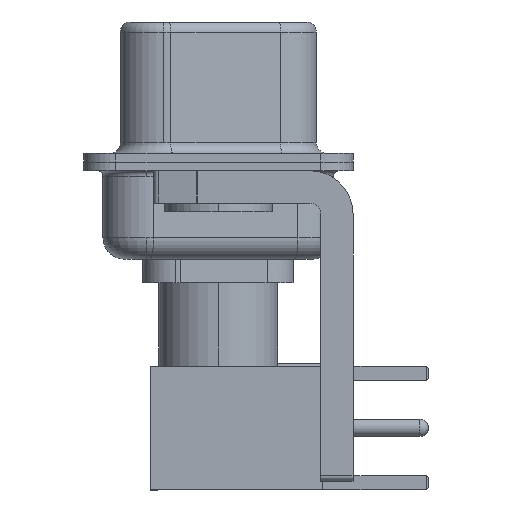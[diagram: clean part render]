
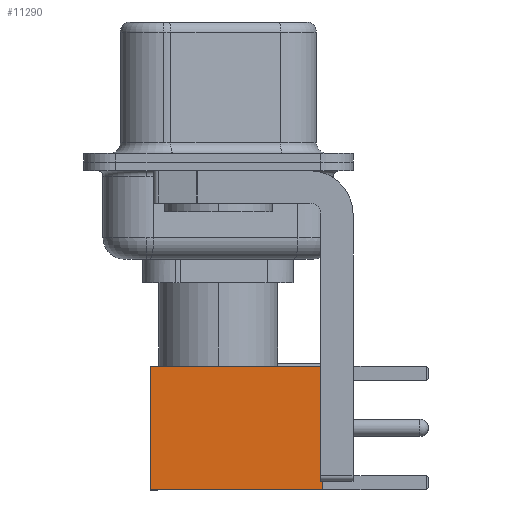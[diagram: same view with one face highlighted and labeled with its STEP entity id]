
A CAD part, left-side view. The second image highlights one B-rep face of the part: STEP entity #11290.
In plain terms, the highlighted face is planar.
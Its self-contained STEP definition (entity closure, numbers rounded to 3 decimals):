
#524 = CARTESIAN_POINT ( 'NONE',  ( 0., 2.875, 8. ) ) ;
#756 = EDGE_CURVE ( 'NONE', #16886, #11554, #18207, .T. ) ;
#2375 = AXIS2_PLACEMENT_3D ( 'NONE', #16512, #8999, #18196 ) ;
#4478 = PLANE ( 'NONE',  #2375 ) ;
#4785 = CARTESIAN_POINT ( 'NONE',  ( -2.875, 2.875, 0. ) ) ;
#5215 = LINE ( 'NONE', #524, #28348 ) ;
#5266 = CARTESIAN_POINT ( 'NONE',  ( 2.875, 2.875, 0. ) ) ;
#6453 = EDGE_CURVE ( 'NONE', #27923, #16886, #5215, .T. ) ;
#6469 = VECTOR ( 'NONE', #14105, 1000. ) ;
#7337 = FACE_OUTER_BOUND ( 'NONE', #20268, .T. ) ;
#8255 = CARTESIAN_POINT ( 'NONE',  ( 0., 2.875, 0. ) ) ;
#8999 = DIRECTION ( 'NONE',  ( 0., 1., 0. ) ) ;
#10598 = VECTOR ( 'NONE', #17143, 1000. ) ;
#11284 = VERTEX_POINT ( 'NONE', #20448 ) ;
#11290 = ADVANCED_FACE ( 'NONE', ( #7337 ), #4478, .T. ) ;
#11554 = VERTEX_POINT ( 'NONE', #23455 ) ;
#11749 = DIRECTION ( 'NONE',  ( 0., 0., -1. ) ) ;
#12223 = EDGE_CURVE ( 'NONE', #11284, #11554, #12325, .T. ) ;
#12325 = LINE ( 'NONE', #8255, #10598 ) ;
#14105 = DIRECTION ( 'NONE',  ( 0., 0., -1. ) ) ;
#14378 = DIRECTION ( 'NONE',  ( -1., 0., 0. ) ) ;
#16512 = CARTESIAN_POINT ( 'NONE',  ( 2.875, 2.875, 0. ) ) ;
#16886 = VERTEX_POINT ( 'NONE', #20046 ) ;
#17143 = DIRECTION ( 'NONE',  ( -1., 0., 0. ) ) ;
#18196 = DIRECTION ( 'NONE',  ( 0., 0., 1. ) ) ;
#18207 = LINE ( 'NONE', #4785, #6469 ) ;
#19297 = ORIENTED_EDGE ( 'NONE', *, *, #27304, .T. ) ;
#20046 = CARTESIAN_POINT ( 'NONE',  ( -2.875, 2.875, 8. ) ) ;
#20077 = ORIENTED_EDGE ( 'NONE', *, *, #756, .F. ) ;
#20268 = EDGE_LOOP ( 'NONE', ( #19297, #24986, #20077, #25475 ) ) ;
#20448 = CARTESIAN_POINT ( 'NONE',  ( 2.875, 2.875, 0. ) ) ;
#22421 = VECTOR ( 'NONE', #11749, 1000. ) ;
#23034 = CARTESIAN_POINT ( 'NONE',  ( 2.875, 2.875, 8. ) ) ;
#23362 = LINE ( 'NONE', #5266, #22421 ) ;
#23455 = CARTESIAN_POINT ( 'NONE',  ( -2.875, 2.875, 0. ) ) ;
#24986 = ORIENTED_EDGE ( 'NONE', *, *, #12223, .T. ) ;
#25475 = ORIENTED_EDGE ( 'NONE', *, *, #6453, .F. ) ;
#27304 = EDGE_CURVE ( 'NONE', #27923, #11284, #23362, .T. ) ;
#27923 = VERTEX_POINT ( 'NONE', #23034 ) ;
#28348 = VECTOR ( 'NONE', #14378, 1000. ) ;
